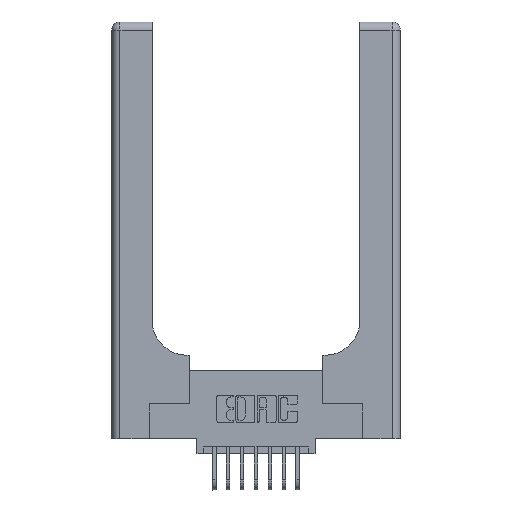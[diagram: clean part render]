
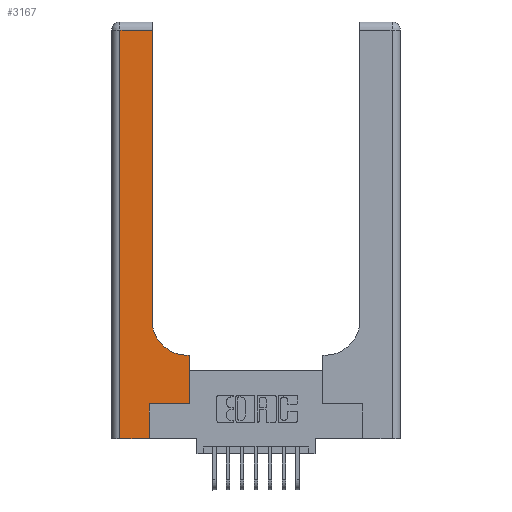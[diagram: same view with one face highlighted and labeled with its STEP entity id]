
A CAD part, top view. The second image highlights one B-rep face of the part: STEP entity #3167.
In plain terms, the highlighted planar face has unit normal (0, 0, 1).
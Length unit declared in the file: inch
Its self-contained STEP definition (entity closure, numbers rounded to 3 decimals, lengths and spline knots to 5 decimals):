
#115 = VERTEX_POINT ( 'NONE', #15117 ) ;
#269 = VECTOR ( 'NONE', #1122, 39.37008 ) ;
#560 = VERTEX_POINT ( 'NONE', #4947 ) ;
#660 = VERTEX_POINT ( 'NONE', #10732 ) ;
#777 = CARTESIAN_POINT ( 'NONE',  ( 0.269, 0.25, 0.37 ) ) ;
#1122 = DIRECTION ( 'NONE',  ( 0., 1., 0. ) ) ;
#1458 = EDGE_CURVE ( 'NONE', #6045, #10531, #7535, .T. ) ;
#1622 = ORIENTED_EDGE ( 'NONE', *, *, #2380, .T. ) ;
#1691 = CARTESIAN_POINT ( 'NONE',  ( 0.5585, 0.25, 0.37 ) ) ;
#1852 = DIRECTION ( 'NONE',  ( -1., 0., 0. ) ) ;
#2019 = ORIENTED_EDGE ( 'NONE', *, *, #14757, .T. ) ;
#2205 = LINE ( 'NONE', #7246, #4640 ) ;
#2230 = EDGE_CURVE ( 'NONE', #15077, #5101, #10481, .T. ) ;
#2328 = CIRCLE ( 'NONE', #6944, 0.25 ) ;
#2380 = EDGE_CURVE ( 'NONE', #560, #6045, #5024, .T. ) ;
#2469 = ORIENTED_EDGE ( 'NONE', *, *, #13980, .T. ) ;
#2514 = ORIENTED_EDGE ( 'NONE', *, *, #10131, .T. ) ;
#2529 = CARTESIAN_POINT ( 'NONE',  ( 0., 3., 0.37 ) ) ;
#2557 = DIRECTION ( 'NONE',  ( 0., 1., 0. ) ) ;
#2731 = ORIENTED_EDGE ( 'NONE', *, *, #13878, .T. ) ;
#3095 = ORIENTED_EDGE ( 'NONE', *, *, #2230, .T. ) ;
#3167 = ADVANCED_FACE ( 'NONE', ( #7295 ), #13236, .F. ) ;
#3241 = ORIENTED_EDGE ( 'NONE', *, *, #11891, .T. ) ;
#3497 = ORIENTED_EDGE ( 'NONE', *, *, #1458, .T. ) ;
#3844 = LINE ( 'NONE', #13630, #9489 ) ;
#3885 = LINE ( 'NONE', #8389, #269 ) ;
#3988 = CARTESIAN_POINT ( 'NONE',  ( 0.269, 0., 0.37 ) ) ;
#4098 = VECTOR ( 'NONE', #13402, 39.37008 ) ;
#4108 = DIRECTION ( 'NONE',  ( 1., 0., 0. ) ) ;
#4163 = CARTESIAN_POINT ( 'NONE',  ( 0.2915, 0.6, 0.37 ) ) ;
#4290 = VECTOR ( 'NONE', #15342, 39.37008 ) ;
#4397 = CARTESIAN_POINT ( 'NONE',  ( 0.5415, 0.85, 0.37 ) ) ;
#4551 = VECTOR ( 'NONE', #2557, 39.37008 ) ;
#4640 = VECTOR ( 'NONE', #4843, 39.37008 ) ;
#4679 = CARTESIAN_POINT ( 'NONE',  ( 0.06, 3., 0.37 ) ) ;
#4843 = DIRECTION ( 'NONE',  ( 1., 0., 0. ) ) ;
#4884 = LINE ( 'NONE', #4163, #8125 ) ;
#4947 = CARTESIAN_POINT ( 'NONE',  ( 0.2915, 2.94, 0.37 ) ) ;
#4989 = CARTESIAN_POINT ( 'NONE',  ( 0.06, 0., 0.37 ) ) ;
#5024 = LINE ( 'NONE', #10270, #11753 ) ;
#5101 = VERTEX_POINT ( 'NONE', #777 ) ;
#5625 = DIRECTION ( 'NONE',  ( 1., 0., 0. ) ) ;
#6045 = VERTEX_POINT ( 'NONE', #6257 ) ;
#6166 = DIRECTION ( 'NONE',  ( 0., 0., -1. ) ) ;
#6257 = CARTESIAN_POINT ( 'NONE',  ( 0.06, 2.94, 0.37 ) ) ;
#6944 = AXIS2_PLACEMENT_3D ( 'NONE', #4397, #12727, #5625 ) ;
#7246 = CARTESIAN_POINT ( 'NONE',  ( 0., 0., 0.37 ) ) ;
#7295 = FACE_OUTER_BOUND ( 'NONE', #7530, .T. ) ;
#7530 = EDGE_LOOP ( 'NONE', ( #13907, #1622, #3497, #3241, #3095, #2731, #2019, #2514, #2469 ) ) ;
#7535 = LINE ( 'NONE', #4679, #4290 ) ;
#7623 = VERTEX_POINT ( 'NONE', #10557 ) ;
#8125 = VECTOR ( 'NONE', #12488, 39.37008 ) ;
#8322 = VERTEX_POINT ( 'NONE', #1691 ) ;
#8389 = CARTESIAN_POINT ( 'NONE',  ( 0.2915, 3., 0.37 ) ) ;
#8531 = CARTESIAN_POINT ( 'NONE',  ( 0.5585, 0.25, 0.37 ) ) ;
#9489 = VECTOR ( 'NONE', #4108, 39.37008 ) ;
#9967 = AXIS2_PLACEMENT_3D ( 'NONE', #2529, #6166, #14385 ) ;
#10131 = EDGE_CURVE ( 'NONE', #115, #660, #4884, .T. ) ;
#10270 = CARTESIAN_POINT ( 'NONE',  ( 0., 2.94, 0.37 ) ) ;
#10375 = CARTESIAN_POINT ( 'NONE',  ( 0.269, 0., 0.37 ) ) ;
#10481 = LINE ( 'NONE', #3988, #4098 ) ;
#10531 = VERTEX_POINT ( 'NONE', #4989 ) ;
#10557 = CARTESIAN_POINT ( 'NONE',  ( 0.2915, 0.85, 0.37 ) ) ;
#10732 = CARTESIAN_POINT ( 'NONE',  ( 0.5415, 0.6, 0.37 ) ) ;
#11753 = VECTOR ( 'NONE', #1852, 39.37008 ) ;
#11891 = EDGE_CURVE ( 'NONE', #10531, #15077, #2205, .T. ) ;
#12425 = EDGE_CURVE ( 'NONE', #7623, #560, #3885, .T. ) ;
#12488 = DIRECTION ( 'NONE',  ( -1., 0., 0. ) ) ;
#12727 = DIRECTION ( 'NONE',  ( 0., 0., -1. ) ) ;
#13236 = PLANE ( 'NONE',  #9967 ) ;
#13402 = DIRECTION ( 'NONE',  ( 0., 1., 0. ) ) ;
#13630 = CARTESIAN_POINT ( 'NONE',  ( 0.269, 0.25, 0.37 ) ) ;
#13878 = EDGE_CURVE ( 'NONE', #5101, #8322, #3844, .T. ) ;
#13907 = ORIENTED_EDGE ( 'NONE', *, *, #12425, .T. ) ;
#13980 = EDGE_CURVE ( 'NONE', #660, #7623, #2328, .T. ) ;
#13989 = LINE ( 'NONE', #8531, #4551 ) ;
#14385 = DIRECTION ( 'NONE',  ( -1., 0., 0. ) ) ;
#14757 = EDGE_CURVE ( 'NONE', #8322, #115, #13989, .T. ) ;
#15077 = VERTEX_POINT ( 'NONE', #10375 ) ;
#15117 = CARTESIAN_POINT ( 'NONE',  ( 0.5585, 0.6, 0.37 ) ) ;
#15342 = DIRECTION ( 'NONE',  ( 0., -1., 0. ) ) ;
